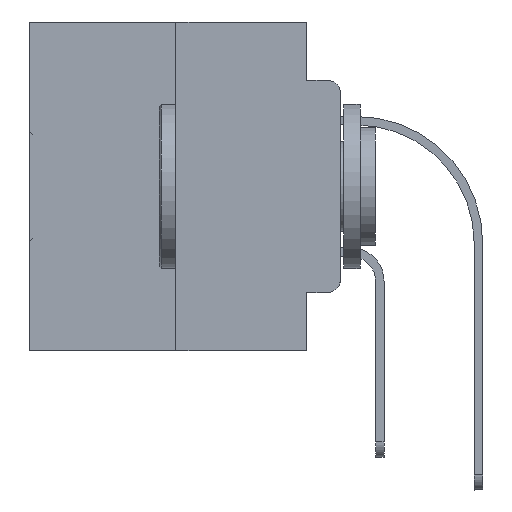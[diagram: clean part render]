
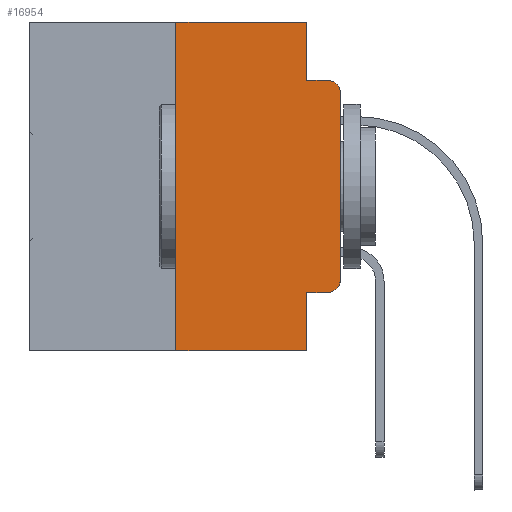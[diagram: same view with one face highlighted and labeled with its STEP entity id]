
A CAD part, left-side view. The second image highlights one B-rep face of the part: STEP entity #16954.
In plain terms, the highlighted planar face has unit normal (-1, 0, 0).
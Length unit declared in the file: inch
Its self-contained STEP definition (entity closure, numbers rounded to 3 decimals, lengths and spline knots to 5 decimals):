
#30 = DIRECTION ( 'NONE',  ( 0., 0., -1. ) ) ;
#198 = CARTESIAN_POINT ( 'NONE',  ( 0., 0.02, -0.3915 ) ) ;
#1006 = CARTESIAN_POINT ( 'NONE',  ( 0., 0.051, -0.0885 ) ) ;
#2270 = ORIENTED_EDGE ( 'NONE', *, *, #12897, .T. ) ;
#2695 = VECTOR ( 'NONE', #12886, 39.37008 ) ;
#3819 = EDGE_CURVE ( 'NONE', #31061, #17454, #6827, .T. ) ;
#4770 = DIRECTION ( 'NONE',  ( 0., -1., 0. ) ) ;
#5568 = DIRECTION ( 'NONE',  ( 0., -1., 0. ) ) ;
#6138 = VERTEX_POINT ( 'NONE', #21312 ) ;
#6217 = CIRCLE ( 'NONE', #20151, 0.02 ) ;
#6275 = DIRECTION ( 'NONE',  ( -1., 0., 0. ) ) ;
#6423 = EDGE_CURVE ( 'NONE', #6138, #25129, #25826, .T. ) ;
#6476 = FACE_OUTER_BOUND ( 'NONE', #23592, .T. ) ;
#6569 = CIRCLE ( 'NONE', #8797, 0.02 ) ;
#6827 = LINE ( 'NONE', #28505, #12132 ) ;
#7228 = ORIENTED_EDGE ( 'NONE', *, *, #3819, .F. ) ;
#7786 = ORIENTED_EDGE ( 'NONE', *, *, #6423, .T. ) ;
#7799 = LINE ( 'NONE', #25627, #8076 ) ;
#8076 = VECTOR ( 'NONE', #18449, 39.37008 ) ;
#8599 = ORIENTED_EDGE ( 'NONE', *, *, #8883, .T. ) ;
#8797 = AXIS2_PLACEMENT_3D ( 'NONE', #12019, #6275, #14307 ) ;
#8883 = EDGE_CURVE ( 'NONE', #14600, #6138, #6217, .T. ) ;
#9270 = DIRECTION ( 'NONE',  ( 0., 0., -1. ) ) ;
#9499 = EDGE_CURVE ( 'NONE', #17454, #15370, #7799, .T. ) ;
#9759 = LINE ( 'NONE', #20406, #20338 ) ;
#9944 = CARTESIAN_POINT ( 'NONE',  ( 0., 0.051, 0. ) ) ;
#9988 = DIRECTION ( 'NONE',  ( 0., 0., -1. ) ) ;
#10186 = CARTESIAN_POINT ( 'NONE',  ( 0., 0.25, 0. ) ) ;
#10811 = EDGE_CURVE ( 'NONE', #22740, #22250, #15774, .T. ) ;
#11555 = CARTESIAN_POINT ( 'NONE',  ( 0., 0.473, 0. ) ) ;
#12019 = CARTESIAN_POINT ( 'NONE',  ( 0., 0.02, -0.1085 ) ) ;
#12034 = DIRECTION ( 'NONE',  ( 0., -1., 0. ) ) ;
#12132 = VECTOR ( 'NONE', #20098, 39.37008 ) ;
#12886 = DIRECTION ( 'NONE',  ( 0., 0., 1. ) ) ;
#12897 = EDGE_CURVE ( 'NONE', #20981, #14600, #9759, .T. ) ;
#13067 = LINE ( 'NONE', #21449, #18697 ) ;
#13139 = CARTESIAN_POINT ( 'NONE',  ( 0., 0.473, -0.5 ) ) ;
#14307 = DIRECTION ( 'NONE',  ( 0., 0., -1. ) ) ;
#14600 = VERTEX_POINT ( 'NONE', #32595 ) ;
#15047 = LINE ( 'NONE', #30939, #20869 ) ;
#15370 = VERTEX_POINT ( 'NONE', #29055 ) ;
#15774 = LINE ( 'NONE', #13139, #25282 ) ;
#16132 = DIRECTION ( 'NONE',  ( -1., 0., 0. ) ) ;
#16954 = ADVANCED_FACE ( 'NONE', ( #6476 ), #25186, .F. ) ;
#17138 = DIRECTION ( 'NONE',  ( 1., 0., 0. ) ) ;
#17373 = EDGE_CURVE ( 'NONE', #25129, #15370, #6569, .T. ) ;
#17454 = VERTEX_POINT ( 'NONE', #1006 ) ;
#17782 = CARTESIAN_POINT ( 'NONE',  ( 0., 0., 0. ) ) ;
#18449 = DIRECTION ( 'NONE',  ( 0., -1., 0. ) ) ;
#18697 = VECTOR ( 'NONE', #5568, 39.37008 ) ;
#19171 = CARTESIAN_POINT ( 'NONE',  ( 0., 0.051, -0.5 ) ) ;
#20098 = DIRECTION ( 'NONE',  ( 0., 0., -1. ) ) ;
#20151 = AXIS2_PLACEMENT_3D ( 'NONE', #198, #16132, #30 ) ;
#20338 = VECTOR ( 'NONE', #12034, 39.37008 ) ;
#20406 = CARTESIAN_POINT ( 'NONE',  ( 0., 0.051, -0.4115 ) ) ;
#20478 = EDGE_CURVE ( 'NONE', #22740, #22797, #33331, .T. ) ;
#20659 = CARTESIAN_POINT ( 'NONE',  ( 0., 0.25, -0.5 ) ) ;
#20869 = VECTOR ( 'NONE', #9988, 39.37008 ) ;
#20981 = VERTEX_POINT ( 'NONE', #22310 ) ;
#21219 = ORIENTED_EDGE ( 'NONE', *, *, #29273, .F. ) ;
#21312 = CARTESIAN_POINT ( 'NONE',  ( 0., 0., -0.3915 ) ) ;
#21449 = CARTESIAN_POINT ( 'NONE',  ( 0., 0.473, 0. ) ) ;
#22250 = VERTEX_POINT ( 'NONE', #19171 ) ;
#22310 = CARTESIAN_POINT ( 'NONE',  ( 0., 0.051, -0.4115 ) ) ;
#22740 = VERTEX_POINT ( 'NONE', #20659 ) ;
#22797 = VERTEX_POINT ( 'NONE', #10186 ) ;
#23592 = EDGE_LOOP ( 'NONE', ( #7786, #24744, #30918, #7228, #21219, #26720, #25686, #30214, #2270, #8599 ) ) ;
#24744 = ORIENTED_EDGE ( 'NONE', *, *, #17373, .T. ) ;
#25129 = VERTEX_POINT ( 'NONE', #29555 ) ;
#25186 = PLANE ( 'NONE',  #26657 ) ;
#25282 = VECTOR ( 'NONE', #4770, 39.37008 ) ;
#25627 = CARTESIAN_POINT ( 'NONE',  ( 0., 0.051, -0.0885 ) ) ;
#25686 = ORIENTED_EDGE ( 'NONE', *, *, #10811, .T. ) ;
#25826 = LINE ( 'NONE', #17782, #2695 ) ;
#26211 = VECTOR ( 'NONE', #32998, 39.37008 ) ;
#26657 = AXIS2_PLACEMENT_3D ( 'NONE', #11555, #17138, #9270 ) ;
#26720 = ORIENTED_EDGE ( 'NONE', *, *, #20478, .F. ) ;
#28505 = CARTESIAN_POINT ( 'NONE',  ( 0., 0.051, 0. ) ) ;
#28685 = EDGE_CURVE ( 'NONE', #20981, #22250, #15047, .T. ) ;
#29055 = CARTESIAN_POINT ( 'NONE',  ( 0., 0.02, -0.0885 ) ) ;
#29273 = EDGE_CURVE ( 'NONE', #22797, #31061, #13067, .T. ) ;
#29555 = CARTESIAN_POINT ( 'NONE',  ( 0., 0., -0.1085 ) ) ;
#30214 = ORIENTED_EDGE ( 'NONE', *, *, #28685, .F. ) ;
#30918 = ORIENTED_EDGE ( 'NONE', *, *, #9499, .F. ) ;
#30939 = CARTESIAN_POINT ( 'NONE',  ( 0., 0.051, 0. ) ) ;
#31061 = VERTEX_POINT ( 'NONE', #9944 ) ;
#32595 = CARTESIAN_POINT ( 'NONE',  ( 0., 0.02, -0.4115 ) ) ;
#32998 = DIRECTION ( 'NONE',  ( 0., 0., 1. ) ) ;
#33164 = CARTESIAN_POINT ( 'NONE',  ( 0., 0.25, 0. ) ) ;
#33331 = LINE ( 'NONE', #33164, #26211 ) ;
